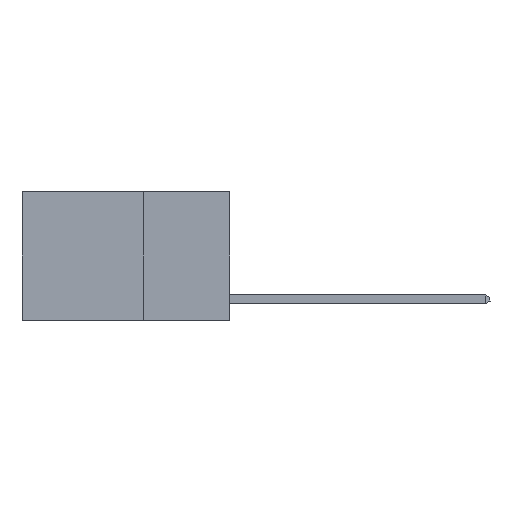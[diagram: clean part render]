
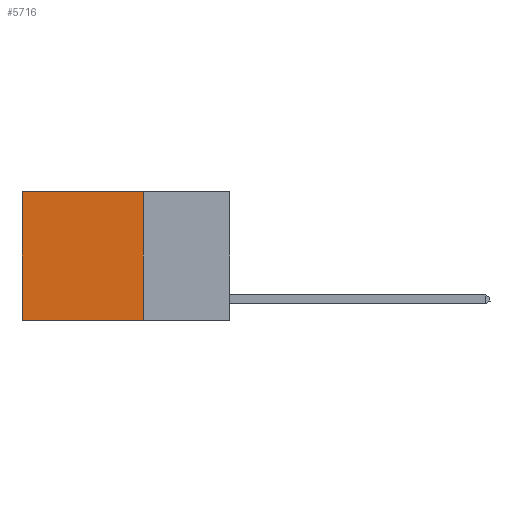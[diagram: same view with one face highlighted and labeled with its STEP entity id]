
A CAD part, left-side view. The second image highlights one B-rep face of the part: STEP entity #5716.
In plain terms, the highlighted planar face has unit normal (-1, 0, 0).
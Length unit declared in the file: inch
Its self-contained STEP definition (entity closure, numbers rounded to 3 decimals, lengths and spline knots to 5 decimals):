
#750 = VERTEX_POINT ( 'NONE', #13263 ) ;
#1712 = ORIENTED_EDGE ( 'NONE', *, *, #20801, .T. ) ;
#1720 = LINE ( 'NONE', #6734, #10268 ) ;
#2148 = EDGE_CURVE ( 'NONE', #750, #4787, #18791, .T. ) ;
#2300 = CARTESIAN_POINT ( 'NONE',  ( 0.2625, 0.25, 0. ) ) ;
#2319 = DIRECTION ( 'NONE',  ( 0., 1., 0. ) ) ;
#2628 = CARTESIAN_POINT ( 'NONE',  ( 0.2625, 0.25, 0. ) ) ;
#4049 = CARTESIAN_POINT ( 'NONE',  ( 0.2625, 0.25, 0. ) ) ;
#4359 = DIRECTION ( 'NONE',  ( 0., 1., 0. ) ) ;
#4787 = VERTEX_POINT ( 'NONE', #6158 ) ;
#4998 = DIRECTION ( 'NONE',  ( 0., 0., -1. ) ) ;
#5713 = EDGE_LOOP ( 'NONE', ( #1712, #6428, #16800, #13417 ) ) ;
#5716 = ADVANCED_FACE ( 'NONE', ( #17298 ), #14292, .F. ) ;
#5737 = DIRECTION ( 'NONE',  ( 1., 0., 0. ) ) ;
#5997 = VECTOR ( 'NONE', #12562, 39.37008 ) ;
#6158 = CARTESIAN_POINT ( 'NONE',  ( 0.2625, 0.6, -0.37 ) ) ;
#6428 = ORIENTED_EDGE ( 'NONE', *, *, #2148, .F. ) ;
#6734 = CARTESIAN_POINT ( 'NONE',  ( 0.2625, 0.6, 0. ) ) ;
#6787 = CARTESIAN_POINT ( 'NONE',  ( 0.2625, 0.6, 0. ) ) ;
#7666 = EDGE_CURVE ( 'NONE', #17032, #9524, #12947, .T. ) ;
#9524 = VERTEX_POINT ( 'NONE', #6787 ) ;
#10268 = VECTOR ( 'NONE', #4998, 39.37008 ) ;
#12461 = AXIS2_PLACEMENT_3D ( 'NONE', #4049, #5737, #17739 ) ;
#12562 = DIRECTION ( 'NONE',  ( 0., 0., -1. ) ) ;
#12947 = LINE ( 'NONE', #2628, #21519 ) ;
#13263 = CARTESIAN_POINT ( 'NONE',  ( 0.2625, 0.25, -0.37 ) ) ;
#13417 = ORIENTED_EDGE ( 'NONE', *, *, #7666, .T. ) ;
#14233 = VECTOR ( 'NONE', #2319, 39.37008 ) ;
#14292 = PLANE ( 'NONE',  #12461 ) ;
#15148 = LINE ( 'NONE', #2300, #5997 ) ;
#15723 = CARTESIAN_POINT ( 'NONE',  ( 0.2625, 0.25, 0. ) ) ;
#16800 = ORIENTED_EDGE ( 'NONE', *, *, #17823, .F. ) ;
#17032 = VERTEX_POINT ( 'NONE', #15723 ) ;
#17298 = FACE_OUTER_BOUND ( 'NONE', #5713, .T. ) ;
#17655 = CARTESIAN_POINT ( 'NONE',  ( 0.2625, 0.25, -0.37 ) ) ;
#17739 = DIRECTION ( 'NONE',  ( 0., 0., -1. ) ) ;
#17823 = EDGE_CURVE ( 'NONE', #17032, #750, #15148, .T. ) ;
#18791 = LINE ( 'NONE', #17655, #14233 ) ;
#20801 = EDGE_CURVE ( 'NONE', #9524, #4787, #1720, .T. ) ;
#21519 = VECTOR ( 'NONE', #4359, 39.37008 ) ;
